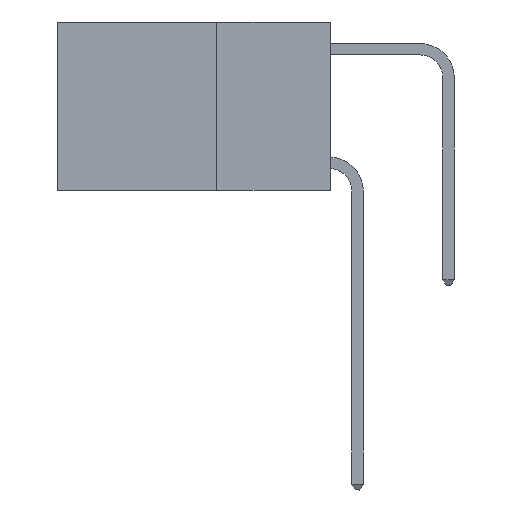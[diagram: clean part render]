
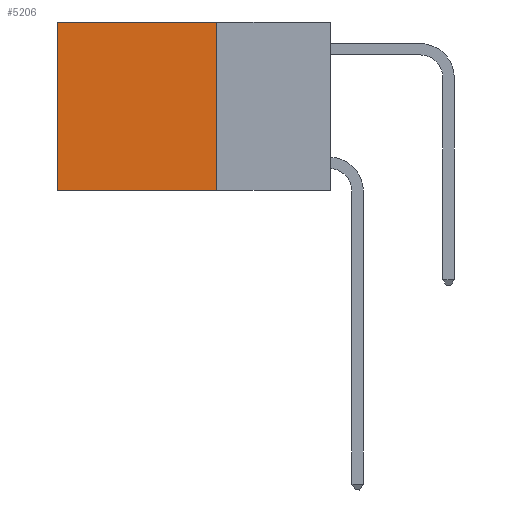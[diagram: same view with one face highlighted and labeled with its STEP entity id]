
A CAD part, left-side view. The second image highlights one B-rep face of the part: STEP entity #5206.
In plain terms, the highlighted planar face has unit normal (-1, 0, 0).
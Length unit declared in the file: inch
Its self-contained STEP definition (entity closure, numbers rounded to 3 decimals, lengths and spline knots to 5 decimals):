
#33 = VERTEX_POINT ( 'NONE', #1599 ) ;
#286 = CARTESIAN_POINT ( 'NONE',  ( 0.2625, 0.6, 0. ) ) ;
#632 = VERTEX_POINT ( 'NONE', #286 ) ;
#843 = LINE ( 'NONE', #9175, #4577 ) ;
#1066 = EDGE_LOOP ( 'NONE', ( #2982, #15660, #16985, #17544 ) ) ;
#1599 = CARTESIAN_POINT ( 'NONE',  ( 0.2625, 0.6, -0.37 ) ) ;
#2041 = AXIS2_PLACEMENT_3D ( 'NONE', #16827, #18589, #9072 ) ;
#2684 = EDGE_CURVE ( 'NONE', #632, #33, #13373, .T. ) ;
#2807 = CARTESIAN_POINT ( 'NONE',  ( 0.2625, 0.25, 0. ) ) ;
#2982 = ORIENTED_EDGE ( 'NONE', *, *, #2684, .T. ) ;
#3553 = CARTESIAN_POINT ( 'NONE',  ( 0.2625, 0.6, 0. ) ) ;
#3680 = DIRECTION ( 'NONE',  ( 0., 1., 0. ) ) ;
#4415 = DIRECTION ( 'NONE',  ( 0., 0., -1. ) ) ;
#4577 = VECTOR ( 'NONE', #18483, 39.37008 ) ;
#4595 = LINE ( 'NONE', #2807, #5334 ) ;
#4818 = VECTOR ( 'NONE', #3680, 39.37008 ) ;
#5206 = ADVANCED_FACE ( 'NONE', ( #6903 ), #5671, .F. ) ;
#5334 = VECTOR ( 'NONE', #4415, 39.37008 ) ;
#5671 = PLANE ( 'NONE',  #2041 ) ;
#6065 = EDGE_CURVE ( 'NONE', #13748, #632, #15244, .T. ) ;
#6903 = FACE_OUTER_BOUND ( 'NONE', #1066, .T. ) ;
#9072 = DIRECTION ( 'NONE',  ( 0., 0., -1. ) ) ;
#9175 = CARTESIAN_POINT ( 'NONE',  ( 0.2625, 0.25, -0.37 ) ) ;
#9333 = CARTESIAN_POINT ( 'NONE',  ( 0.2625, 0.25, 0. ) ) ;
#10063 = CARTESIAN_POINT ( 'NONE',  ( 0.2625, 0.25, 0. ) ) ;
#11277 = DIRECTION ( 'NONE',  ( 0., 0., -1. ) ) ;
#13373 = LINE ( 'NONE', #3553, #16613 ) ;
#13748 = VERTEX_POINT ( 'NONE', #9333 ) ;
#13794 = EDGE_CURVE ( 'NONE', #13748, #17192, #4595, .T. ) ;
#14281 = EDGE_CURVE ( 'NONE', #17192, #33, #843, .T. ) ;
#15244 = LINE ( 'NONE', #10063, #4818 ) ;
#15660 = ORIENTED_EDGE ( 'NONE', *, *, #14281, .F. ) ;
#16613 = VECTOR ( 'NONE', #11277, 39.37008 ) ;
#16827 = CARTESIAN_POINT ( 'NONE',  ( 0.2625, 0.25, 0. ) ) ;
#16985 = ORIENTED_EDGE ( 'NONE', *, *, #13794, .F. ) ;
#17192 = VERTEX_POINT ( 'NONE', #17663 ) ;
#17544 = ORIENTED_EDGE ( 'NONE', *, *, #6065, .T. ) ;
#17663 = CARTESIAN_POINT ( 'NONE',  ( 0.2625, 0.25, -0.37 ) ) ;
#18483 = DIRECTION ( 'NONE',  ( 0., 1., 0. ) ) ;
#18589 = DIRECTION ( 'NONE',  ( 1., 0., 0. ) ) ;
